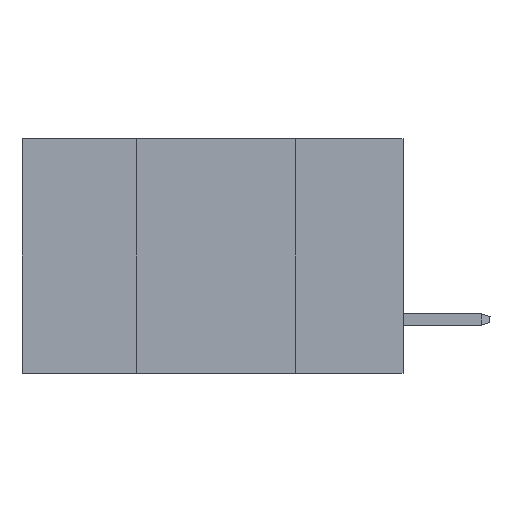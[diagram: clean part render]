
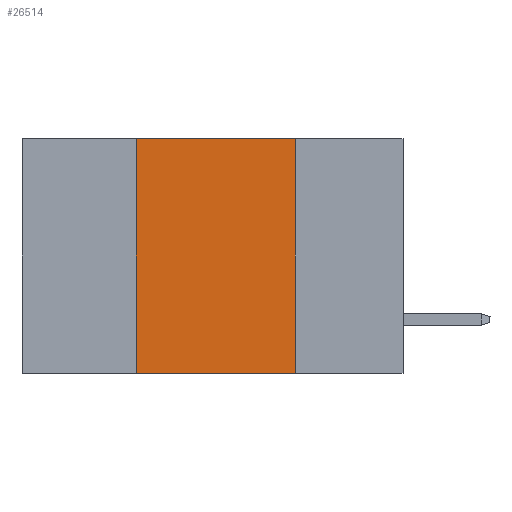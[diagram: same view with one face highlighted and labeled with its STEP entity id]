
A CAD part, left-side view. The second image highlights one B-rep face of the part: STEP entity #26514.
In plain terms, the highlighted planar face has unit normal (-1, 0, 0).
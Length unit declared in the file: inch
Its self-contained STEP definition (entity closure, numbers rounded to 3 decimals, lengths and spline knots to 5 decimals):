
#466 = DIRECTION ( 'NONE',  ( 1., 0., 0. ) ) ;
#2314 = CARTESIAN_POINT ( 'NONE',  ( 0., 0.42, 0. ) ) ;
#3145 = ORIENTED_EDGE ( 'NONE', *, *, #13265, .T. ) ;
#5411 = LINE ( 'NONE', #2314, #14279 ) ;
#5753 = EDGE_CURVE ( 'NONE', #38052, #38075, #5411, .T. ) ;
#6177 = DIRECTION ( 'NONE',  ( 0., -1., 0. ) ) ;
#6836 = CARTESIAN_POINT ( 'NONE',  ( 0., 0.17, 0. ) ) ;
#6856 = ORIENTED_EDGE ( 'NONE', *, *, #41918, .F. ) ;
#9020 = EDGE_LOOP ( 'NONE', ( #6856, #33587, #11073, #3145 ) ) ;
#11073 = ORIENTED_EDGE ( 'NONE', *, *, #5753, .F. ) ;
#11092 = VERTEX_POINT ( 'NONE', #26324 ) ;
#13052 = CARTESIAN_POINT ( 'NONE',  ( 0., 0.6, 0. ) ) ;
#13265 = EDGE_CURVE ( 'NONE', #38052, #39121, #24388, .T. ) ;
#14279 = VECTOR ( 'NONE', #23043, 39.37008 ) ;
#14381 = VECTOR ( 'NONE', #30953, 39.37008 ) ;
#16972 = DIRECTION ( 'NONE',  ( 0., 0., -1. ) ) ;
#17217 = FACE_OUTER_BOUND ( 'NONE', #9020, .T. ) ;
#17488 = LINE ( 'NONE', #34480, #14381 ) ;
#20711 = AXIS2_PLACEMENT_3D ( 'NONE', #13052, #466, #27383 ) ;
#21500 = VECTOR ( 'NONE', #6177, 39.37008 ) ;
#23043 = DIRECTION ( 'NONE',  ( 0., 0., 1. ) ) ;
#24388 = LINE ( 'NONE', #39690, #21500 ) ;
#24391 = VECTOR ( 'NONE', #16972, 39.37008 ) ;
#26179 = EDGE_CURVE ( 'NONE', #38075, #11092, #17488, .T. ) ;
#26324 = CARTESIAN_POINT ( 'NONE',  ( 0., 0.17, 0. ) ) ;
#26514 = ADVANCED_FACE ( 'NONE', ( #17217 ), #30689, .F. ) ;
#27383 = DIRECTION ( 'NONE',  ( 0., 0., -1. ) ) ;
#29947 = CARTESIAN_POINT ( 'NONE',  ( 0., 0.42, -0.37 ) ) ;
#30689 = PLANE ( 'NONE',  #20711 ) ;
#30953 = DIRECTION ( 'NONE',  ( 0., -1., 0. ) ) ;
#33464 = CARTESIAN_POINT ( 'NONE',  ( 0., 0.42, 0. ) ) ;
#33587 = ORIENTED_EDGE ( 'NONE', *, *, #26179, .F. ) ;
#34398 = LINE ( 'NONE', #6836, #24391 ) ;
#34480 = CARTESIAN_POINT ( 'NONE',  ( 0., 0.6, 0. ) ) ;
#38052 = VERTEX_POINT ( 'NONE', #29947 ) ;
#38075 = VERTEX_POINT ( 'NONE', #33464 ) ;
#39121 = VERTEX_POINT ( 'NONE', #41195 ) ;
#39690 = CARTESIAN_POINT ( 'NONE',  ( 0., 0.6, -0.37 ) ) ;
#41195 = CARTESIAN_POINT ( 'NONE',  ( 0., 0.17, -0.37 ) ) ;
#41918 = EDGE_CURVE ( 'NONE', #11092, #39121, #34398, .T. ) ;
